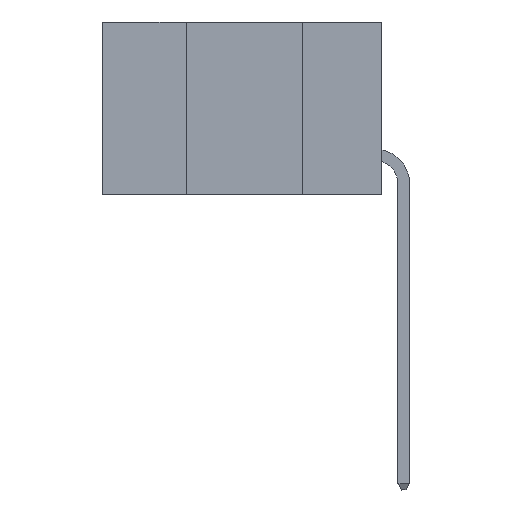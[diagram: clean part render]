
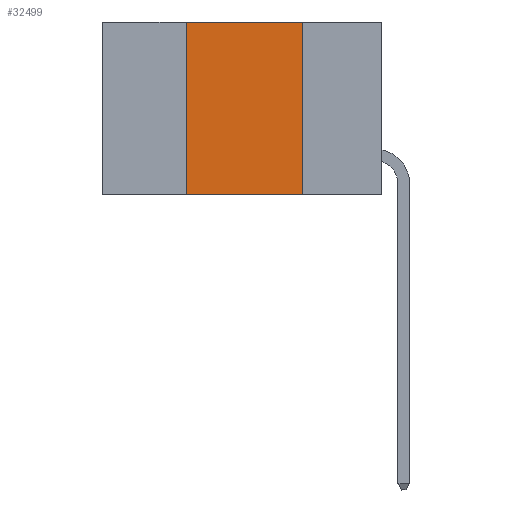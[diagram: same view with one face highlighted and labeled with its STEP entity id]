
A CAD part, left-side view. The second image highlights one B-rep face of the part: STEP entity #32499.
In plain terms, the highlighted planar face has unit normal (-1, 0, 0).
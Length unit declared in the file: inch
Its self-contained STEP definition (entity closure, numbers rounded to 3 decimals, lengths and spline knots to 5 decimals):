
#2849 = VERTEX_POINT ( 'NONE', #14400 ) ;
#3452 = CARTESIAN_POINT ( 'NONE',  ( 0., 0.6, 0. ) ) ;
#3692 = CARTESIAN_POINT ( 'NONE',  ( 0., 0.17, -0.37 ) ) ;
#3783 = CARTESIAN_POINT ( 'NONE',  ( 0., 0.6, 0. ) ) ;
#3932 = VERTEX_POINT ( 'NONE', #3692 ) ;
#4110 = CARTESIAN_POINT ( 'NONE',  ( 0., 0.42, -0.37 ) ) ;
#4795 = VERTEX_POINT ( 'NONE', #4110 ) ;
#8211 = VECTOR ( 'NONE', #18040, 39.37008 ) ;
#9404 = VECTOR ( 'NONE', #20982, 39.37008 ) ;
#10184 = EDGE_CURVE ( 'NONE', #16876, #3932, #40598, .T. ) ;
#10910 = EDGE_CURVE ( 'NONE', #4795, #3932, #37172, .T. ) ;
#10985 = LINE ( 'NONE', #3783, #28054 ) ;
#11217 = EDGE_CURVE ( 'NONE', #2849, #16876, #10985, .T. ) ;
#13147 = DIRECTION ( 'NONE',  ( 0., 0., -1. ) ) ;
#13621 = DIRECTION ( 'NONE',  ( 0., -1., 0. ) ) ;
#14400 = CARTESIAN_POINT ( 'NONE',  ( 0., 0.42, 0. ) ) ;
#15005 = ORIENTED_EDGE ( 'NONE', *, *, #10184, .F. ) ;
#15359 = CARTESIAN_POINT ( 'NONE',  ( 0., 0.42, 0. ) ) ;
#16596 = FACE_OUTER_BOUND ( 'NONE', #23280, .T. ) ;
#16876 = VERTEX_POINT ( 'NONE', #29980 ) ;
#17580 = VECTOR ( 'NONE', #31076, 39.37008 ) ;
#18040 = DIRECTION ( 'NONE',  ( 0., 0., 1. ) ) ;
#18126 = EDGE_CURVE ( 'NONE', #4795, #2849, #25281, .T. ) ;
#19689 = ORIENTED_EDGE ( 'NONE', *, *, #18126, .F. ) ;
#20982 = DIRECTION ( 'NONE',  ( 0., 0., -1. ) ) ;
#23280 = EDGE_LOOP ( 'NONE', ( #15005, #23281, #19689, #40256 ) ) ;
#23281 = ORIENTED_EDGE ( 'NONE', *, *, #11217, .F. ) ;
#24189 = CARTESIAN_POINT ( 'NONE',  ( 0., 0.6, -0.37 ) ) ;
#25281 = LINE ( 'NONE', #15359, #8211 ) ;
#28054 = VECTOR ( 'NONE', #13621, 39.37008 ) ;
#29980 = CARTESIAN_POINT ( 'NONE',  ( 0., 0.17, 0. ) ) ;
#30558 = CARTESIAN_POINT ( 'NONE',  ( 0., 0.17, 0. ) ) ;
#31076 = DIRECTION ( 'NONE',  ( 0., -1., 0. ) ) ;
#32004 = AXIS2_PLACEMENT_3D ( 'NONE', #3452, #32417, #13147 ) ;
#32417 = DIRECTION ( 'NONE',  ( 1., 0., 0. ) ) ;
#32499 = ADVANCED_FACE ( 'NONE', ( #16596 ), #35087, .F. ) ;
#35087 = PLANE ( 'NONE',  #32004 ) ;
#37172 = LINE ( 'NONE', #24189, #17580 ) ;
#40256 = ORIENTED_EDGE ( 'NONE', *, *, #10910, .T. ) ;
#40598 = LINE ( 'NONE', #30558, #9404 ) ;
